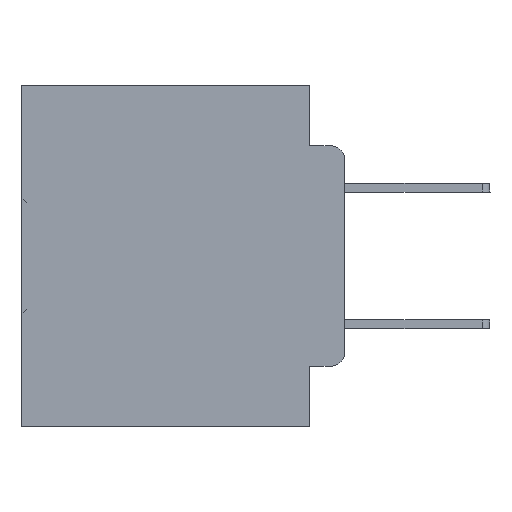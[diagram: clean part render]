
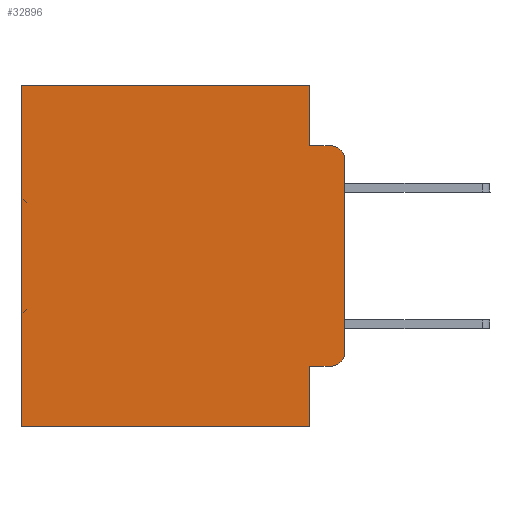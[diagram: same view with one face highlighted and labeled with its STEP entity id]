
A CAD part, left-side view. The second image highlights one B-rep face of the part: STEP entity #32896.
In plain terms, the highlighted planar face has unit normal (-1, 0, 0).
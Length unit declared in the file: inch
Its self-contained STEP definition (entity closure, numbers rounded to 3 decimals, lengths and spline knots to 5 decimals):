
#196 = DIRECTION ( 'NONE',  ( 0., 0., -1. ) ) ;
#233 = DIRECTION ( 'NONE',  ( 0., 0., -1. ) ) ;
#788 = DIRECTION ( 'NONE',  ( 0., 1., 0. ) ) ;
#1254 = CARTESIAN_POINT ( 'NONE',  ( 0.298, 0.051, 0. ) ) ;
#1360 = ORIENTED_EDGE ( 'NONE', *, *, #17315, .T. ) ;
#1808 = DIRECTION ( 'NONE',  ( 0., -1., 0. ) ) ;
#2044 = DIRECTION ( 'NONE',  ( 0., 0., -1. ) ) ;
#3721 = EDGE_CURVE ( 'NONE', #18429, #34117, #25014, .T. ) ;
#4820 = VERTEX_POINT ( 'NONE', #14967 ) ;
#5352 = CARTESIAN_POINT ( 'NONE',  ( 0.298, 0.051, -0.0885 ) ) ;
#5842 = VERTEX_POINT ( 'NONE', #5352 ) ;
#6069 = VECTOR ( 'NONE', #12696, 39.37008 ) ;
#6439 = CIRCLE ( 'NONE', #12158, 0.02 ) ;
#6768 = DIRECTION ( 'NONE',  ( 0., -1., 0. ) ) ;
#7654 = LINE ( 'NONE', #34278, #16403 ) ;
#7885 = VERTEX_POINT ( 'NONE', #18296 ) ;
#8020 = ORIENTED_EDGE ( 'NONE', *, *, #21529, .F. ) ;
#8092 = LINE ( 'NONE', #29866, #27432 ) ;
#8918 = VECTOR ( 'NONE', #22667, 39.37008 ) ;
#9526 = CARTESIAN_POINT ( 'NONE',  ( 0.298, 0.051, -0.0885 ) ) ;
#9616 = DIRECTION ( 'NONE',  ( 0., 0., -1. ) ) ;
#9697 = LINE ( 'NONE', #9526, #24812 ) ;
#9945 = CARTESIAN_POINT ( 'NONE',  ( 0.298, 0.02, -0.4115 ) ) ;
#10083 = CARTESIAN_POINT ( 'NONE',  ( 0.298, 0.02, -0.3915 ) ) ;
#10134 = CARTESIAN_POINT ( 'NONE',  ( 0.298, 0., -0.3915 ) ) ;
#10985 = EDGE_CURVE ( 'NONE', #16561, #34117, #6439, .T. ) ;
#11750 = VECTOR ( 'NONE', #788, 39.37008 ) ;
#11769 = CARTESIAN_POINT ( 'NONE',  ( 0.298, 0.02, -0.0885 ) ) ;
#12158 = AXIS2_PLACEMENT_3D ( 'NONE', #10083, #16720, #196 ) ;
#12696 = DIRECTION ( 'NONE',  ( 0., 0., -1. ) ) ;
#13176 = CARTESIAN_POINT ( 'NONE',  ( 0.298, 0.473, 0. ) ) ;
#13784 = EDGE_CURVE ( 'NONE', #5842, #32706, #9697, .T. ) ;
#13851 = CARTESIAN_POINT ( 'NONE',  ( 0.298, 0.02, -0.1085 ) ) ;
#14204 = ORIENTED_EDGE ( 'NONE', *, *, #10985, .T. ) ;
#14967 = CARTESIAN_POINT ( 'NONE',  ( 0.298, 0.051, -0.4115 ) ) ;
#15199 = LINE ( 'NONE', #34101, #28673 ) ;
#16403 = VECTOR ( 'NONE', #9616, 39.37008 ) ;
#16561 = VERTEX_POINT ( 'NONE', #9945 ) ;
#16720 = DIRECTION ( 'NONE',  ( -1., 0., 0. ) ) ;
#17315 = EDGE_CURVE ( 'NONE', #18429, #32706, #21408, .T. ) ;
#18134 = EDGE_LOOP ( 'NONE', ( #32314, #1360, #29286, #21579, #25293, #32753, #32827, #8020, #25255, #14204 ) ) ;
#18296 = CARTESIAN_POINT ( 'NONE',  ( 0.298, 0.473, 0. ) ) ;
#18429 = VERTEX_POINT ( 'NONE', #30556 ) ;
#19138 = VERTEX_POINT ( 'NONE', #26998 ) ;
#19584 = DIRECTION ( 'NONE',  ( -1., 0., 0. ) ) ;
#21107 = VERTEX_POINT ( 'NONE', #22044 ) ;
#21408 = CIRCLE ( 'NONE', #32863, 0.02 ) ;
#21441 = EDGE_CURVE ( 'NONE', #23531, #5842, #28871, .T. ) ;
#21529 = EDGE_CURVE ( 'NONE', #4820, #19138, #7654, .T. ) ;
#21579 = ORIENTED_EDGE ( 'NONE', *, *, #21441, .F. ) ;
#21750 = DIRECTION ( 'NONE',  ( 0., 1., 0. ) ) ;
#22044 = CARTESIAN_POINT ( 'NONE',  ( 0.298, 0.473, -0.5 ) ) ;
#22333 = LINE ( 'NONE', #33666, #11750 ) ;
#22667 = DIRECTION ( 'NONE',  ( 0., 0., -1. ) ) ;
#23531 = VERTEX_POINT ( 'NONE', #1254 ) ;
#24565 = EDGE_CURVE ( 'NONE', #23531, #7885, #8092, .T. ) ;
#24812 = VECTOR ( 'NONE', #1808, 39.37008 ) ;
#24868 = FACE_OUTER_BOUND ( 'NONE', #18134, .T. ) ;
#25014 = LINE ( 'NONE', #30758, #8918 ) ;
#25255 = ORIENTED_EDGE ( 'NONE', *, *, #27418, .T. ) ;
#25293 = ORIENTED_EDGE ( 'NONE', *, *, #24565, .T. ) ;
#26998 = CARTESIAN_POINT ( 'NONE',  ( 0.298, 0.051, -0.5 ) ) ;
#27234 = CARTESIAN_POINT ( 'NONE',  ( 0.298, 0., 0. ) ) ;
#27418 = EDGE_CURVE ( 'NONE', #4820, #16561, #15199, .T. ) ;
#27432 = VECTOR ( 'NONE', #21750, 39.37008 ) ;
#27719 = DIRECTION ( 'NONE',  ( 0., 0., -1. ) ) ;
#27988 = EDGE_CURVE ( 'NONE', #7885, #21107, #32053, .T. ) ;
#28673 = VECTOR ( 'NONE', #6768, 39.37008 ) ;
#28871 = LINE ( 'NONE', #34455, #6069 ) ;
#29286 = ORIENTED_EDGE ( 'NONE', *, *, #13784, .F. ) ;
#29866 = CARTESIAN_POINT ( 'NONE',  ( 0.298, 0., 0. ) ) ;
#30556 = CARTESIAN_POINT ( 'NONE',  ( 0.298, 0., -0.1085 ) ) ;
#30615 = AXIS2_PLACEMENT_3D ( 'NONE', #27234, #35312, #233 ) ;
#30758 = CARTESIAN_POINT ( 'NONE',  ( 0.298, 0., 0. ) ) ;
#32053 = LINE ( 'NONE', #13176, #32711 ) ;
#32314 = ORIENTED_EDGE ( 'NONE', *, *, #3721, .F. ) ;
#32706 = VERTEX_POINT ( 'NONE', #11769 ) ;
#32711 = VECTOR ( 'NONE', #2044, 39.37008 ) ;
#32753 = ORIENTED_EDGE ( 'NONE', *, *, #27988, .T. ) ;
#32827 = ORIENTED_EDGE ( 'NONE', *, *, #34419, .F. ) ;
#32863 = AXIS2_PLACEMENT_3D ( 'NONE', #13851, #19584, #27719 ) ;
#32896 = ADVANCED_FACE ( 'NONE', ( #24868 ), #35491, .F. ) ;
#33666 = CARTESIAN_POINT ( 'NONE',  ( 0.298, 0., -0.5 ) ) ;
#34101 = CARTESIAN_POINT ( 'NONE',  ( 0.298, 0.051, -0.4115 ) ) ;
#34117 = VERTEX_POINT ( 'NONE', #10134 ) ;
#34278 = CARTESIAN_POINT ( 'NONE',  ( 0.298, 0.051, 0. ) ) ;
#34419 = EDGE_CURVE ( 'NONE', #19138, #21107, #22333, .T. ) ;
#34455 = CARTESIAN_POINT ( 'NONE',  ( 0.298, 0.051, 0. ) ) ;
#35312 = DIRECTION ( 'NONE',  ( 1., 0., 0. ) ) ;
#35491 = PLANE ( 'NONE',  #30615 ) ;
